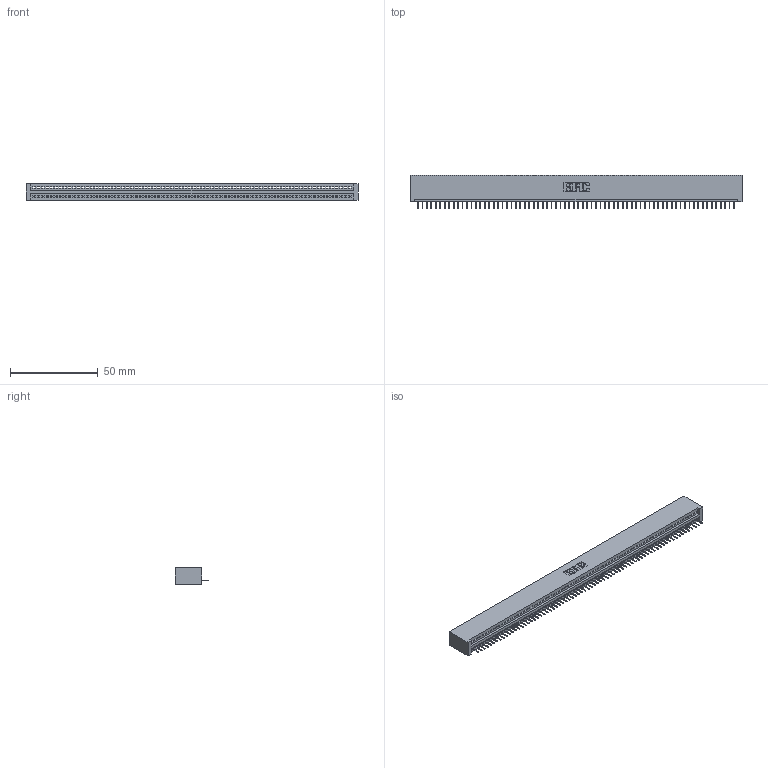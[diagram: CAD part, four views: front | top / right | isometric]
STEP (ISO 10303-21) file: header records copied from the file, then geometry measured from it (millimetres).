
FILE_DESCRIPTION (( 'STEP AP203' ), '1' );
FILE_NAME ('345-072-524-101.STEP', '2019-10-13T04:15:14', ( '' ), ( '' ), 'SwSTEP 2.0', 'SolidWorks 2016', '' );
FILE_SCHEMA (( 'CONFIG_CONTROL_DESIGN' ));
Length unit declared in the file: inch
Products named in the file (3): 345-292-001_345-293-124; 345-072-524-101; 345 Part_No Mounting Lugs
Assembly tree (73 placements, depth 2):
  345-072-524-101
    345 Part_No Mounting Lugs
    345-292-001_345-293-124  x72
Bounding box: 189.48 x 19.35 x 9.4 mm (x, y, z)
Volume: 18543.1 mm3; surface area: 24330.5 mm2
Topology: 73 solids, 73 shells, 4582 faces, 13277 edges, 8562 vertices
Faces by surface type: plane 3388, cylinder 1194
Entity records: 49947 total; most frequent: ORIENTED_EDGE 8662, CARTESIAN_POINT 8656, DIRECTION 7511, EDGE_CURVE 4331, VECTOR 3923, LINE 3923, VERTEX_POINT 2882, AXIS2_PLACEMENT_3D 1794
